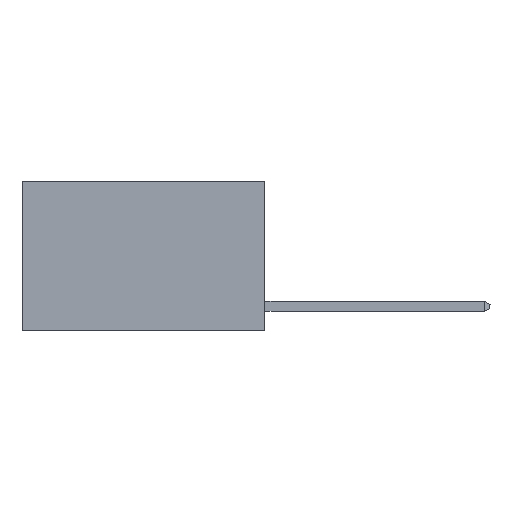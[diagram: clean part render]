
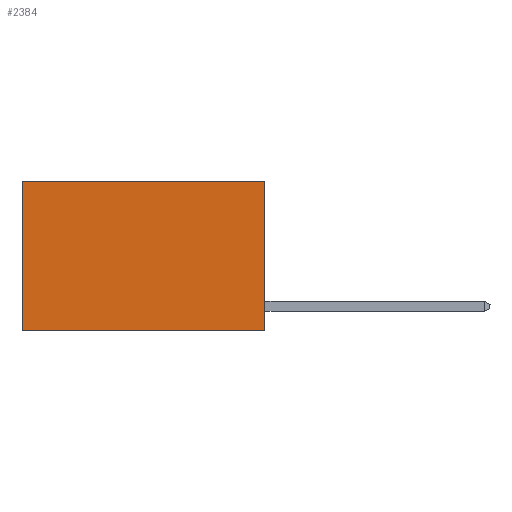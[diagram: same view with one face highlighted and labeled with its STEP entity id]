
A CAD part, left-side view. The second image highlights one B-rep face of the part: STEP entity #2384.
In plain terms, the highlighted planar face has unit normal (-1, 0, 0).
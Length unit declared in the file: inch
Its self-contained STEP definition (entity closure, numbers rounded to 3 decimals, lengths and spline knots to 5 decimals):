
#510 = VERTEX_POINT ( 'NONE', #9401 ) ;
#829 = VERTEX_POINT ( 'NONE', #2801 ) ;
#1696 = CARTESIAN_POINT ( 'NONE',  ( 0.2625, 0., -0.37 ) ) ;
#1840 = VECTOR ( 'NONE', #5903, 39.37008 ) ;
#2135 = AXIS2_PLACEMENT_3D ( 'NONE', #6831, #4931, #2176 ) ;
#2176 = DIRECTION ( 'NONE',  ( 0., 0., -1. ) ) ;
#2384 = ADVANCED_FACE ( 'NONE', ( #9046 ), #11589, .F. ) ;
#2801 = CARTESIAN_POINT ( 'NONE',  ( 0.2625, 0., -0.37 ) ) ;
#4464 = LINE ( 'NONE', #14433, #10859 ) ;
#4931 = DIRECTION ( 'NONE',  ( 1., 0., 0. ) ) ;
#5628 = VECTOR ( 'NONE', #11672, 39.37008 ) ;
#5761 = EDGE_CURVE ( 'NONE', #510, #11983, #4464, .T. ) ;
#5830 = CARTESIAN_POINT ( 'NONE',  ( 0.2625, 0., 0. ) ) ;
#5903 = DIRECTION ( 'NONE',  ( 0., 1., 0. ) ) ;
#6739 = LINE ( 'NONE', #12266, #19635 ) ;
#6831 = CARTESIAN_POINT ( 'NONE',  ( 0.2625, 0., 0. ) ) ;
#7187 = EDGE_CURVE ( 'NONE', #19941, #510, #14879, .T. ) ;
#7583 = ORIENTED_EDGE ( 'NONE', *, *, #7187, .T. ) ;
#8216 = EDGE_CURVE ( 'NONE', #829, #11983, #10987, .T. ) ;
#8313 = CARTESIAN_POINT ( 'NONE',  ( 0.2625, 0.6, -0.37 ) ) ;
#9046 = FACE_OUTER_BOUND ( 'NONE', #17296, .T. ) ;
#9401 = CARTESIAN_POINT ( 'NONE',  ( 0.2625, 0.6, 0. ) ) ;
#10794 = DIRECTION ( 'NONE',  ( 0., 0., -1. ) ) ;
#10859 = VECTOR ( 'NONE', #17657, 39.37008 ) ;
#10929 = ORIENTED_EDGE ( 'NONE', *, *, #20322, .F. ) ;
#10987 = LINE ( 'NONE', #1696, #5628 ) ;
#11520 = ORIENTED_EDGE ( 'NONE', *, *, #5761, .T. ) ;
#11589 = PLANE ( 'NONE',  #2135 ) ;
#11672 = DIRECTION ( 'NONE',  ( 0., 1., 0. ) ) ;
#11983 = VERTEX_POINT ( 'NONE', #8313 ) ;
#12266 = CARTESIAN_POINT ( 'NONE',  ( 0.2625, 0., 0. ) ) ;
#12355 = ORIENTED_EDGE ( 'NONE', *, *, #8216, .F. ) ;
#12893 = CARTESIAN_POINT ( 'NONE',  ( 0.2625, 0., 0. ) ) ;
#14433 = CARTESIAN_POINT ( 'NONE',  ( 0.2625, 0.6, 0. ) ) ;
#14879 = LINE ( 'NONE', #5830, #1840 ) ;
#17296 = EDGE_LOOP ( 'NONE', ( #11520, #12355, #10929, #7583 ) ) ;
#17657 = DIRECTION ( 'NONE',  ( 0., 0., -1. ) ) ;
#19635 = VECTOR ( 'NONE', #10794, 39.37008 ) ;
#19941 = VERTEX_POINT ( 'NONE', #12893 ) ;
#20322 = EDGE_CURVE ( 'NONE', #19941, #829, #6739, .T. ) ;
